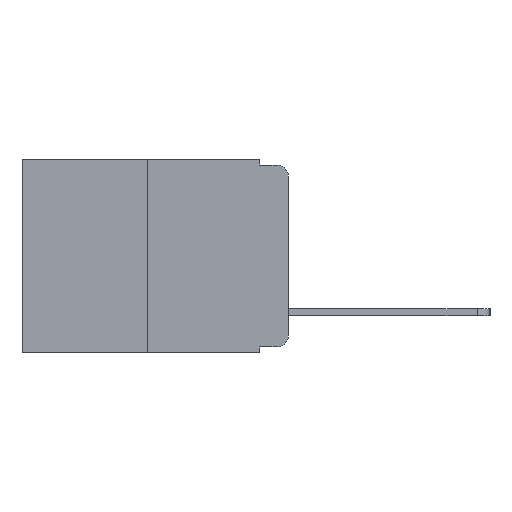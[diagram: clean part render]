
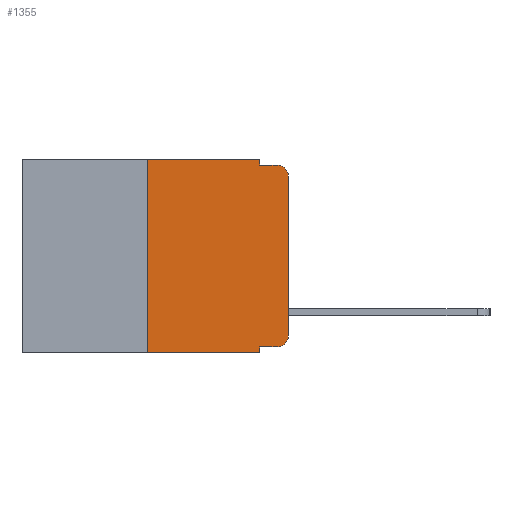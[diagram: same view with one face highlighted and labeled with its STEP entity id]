
A CAD part, left-side view. The second image highlights one B-rep face of the part: STEP entity #1355.
In plain terms, the highlighted planar face has unit normal (-1, 0, 0).
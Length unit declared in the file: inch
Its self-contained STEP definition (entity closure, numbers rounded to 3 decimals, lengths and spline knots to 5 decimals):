
#129 = CARTESIAN_POINT ( 'NONE',  ( 0., 0.051, -0.01 ) ) ;
#455 = VERTEX_POINT ( 'NONE', #19463 ) ;
#535 = CARTESIAN_POINT ( 'NONE',  ( 0., 0.051, 0. ) ) ;
#678 = CARTESIAN_POINT ( 'NONE',  ( 0., 0.25, 0. ) ) ;
#788 = CARTESIAN_POINT ( 'NONE',  ( 0., 0.02, -0.01 ) ) ;
#985 = AXIS2_PLACEMENT_3D ( 'NONE', #14498, #14367, #14458 ) ;
#998 = EDGE_CURVE ( 'NONE', #8953, #3451, #9735, .T. ) ;
#1194 = EDGE_CURVE ( 'NONE', #14783, #3736, #15493, .T. ) ;
#1355 = ADVANCED_FACE ( 'NONE', ( #13234 ), #6686, .F. ) ;
#1556 = VECTOR ( 'NONE', #4362, 39.37008 ) ;
#1994 = EDGE_CURVE ( 'NONE', #14861, #8953, #7348, .T. ) ;
#2044 = LINE ( 'NONE', #19117, #1556 ) ;
#3074 = LINE ( 'NONE', #5772, #10851 ) ;
#3287 = CIRCLE ( 'NONE', #14820, 0.02 ) ;
#3451 = VERTEX_POINT ( 'NONE', #788 ) ;
#3714 = CARTESIAN_POINT ( 'NONE',  ( 0., 0.473, -0.343 ) ) ;
#3736 = VERTEX_POINT ( 'NONE', #535 ) ;
#3832 = CARTESIAN_POINT ( 'NONE',  ( 0., 0.25, 0. ) ) ;
#3848 = VERTEX_POINT ( 'NONE', #13475 ) ;
#4027 = EDGE_CURVE ( 'NONE', #13659, #14783, #7723, .T. ) ;
#4066 = ORIENTED_EDGE ( 'NONE', *, *, #13524, .T. ) ;
#4362 = DIRECTION ( 'NONE',  ( 0., 0., -1. ) ) ;
#4597 = DIRECTION ( 'NONE',  ( -1., 0., 0. ) ) ;
#5683 = DIRECTION ( 'NONE',  ( 0., 0., 1. ) ) ;
#5772 = CARTESIAN_POINT ( 'NONE',  ( 0., 0.051, 0. ) ) ;
#6074 = ORIENTED_EDGE ( 'NONE', *, *, #18397, .F. ) ;
#6305 = VECTOR ( 'NONE', #12080, 39.37008 ) ;
#6686 = PLANE ( 'NONE',  #12114 ) ;
#6854 = VECTOR ( 'NONE', #5683, 39.37008 ) ;
#7272 = ORIENTED_EDGE ( 'NONE', *, *, #1194, .F. ) ;
#7284 = CARTESIAN_POINT ( 'NONE',  ( 0., 0., -0.313 ) ) ;
#7305 = LINE ( 'NONE', #14940, #6305 ) ;
#7348 = LINE ( 'NONE', #14639, #6854 ) ;
#7643 = CARTESIAN_POINT ( 'NONE',  ( 0., 0.051, -0.333 ) ) ;
#7723 = LINE ( 'NONE', #3832, #15604 ) ;
#8248 = CARTESIAN_POINT ( 'NONE',  ( 0., 0.473, 0. ) ) ;
#8554 = LINE ( 'NONE', #3714, #13025 ) ;
#8698 = CARTESIAN_POINT ( 'NONE',  ( 0., 0.25, -0.343 ) ) ;
#8895 = ORIENTED_EDGE ( 'NONE', *, *, #18286, .F. ) ;
#8952 = DIRECTION ( 'NONE',  ( 0., -1., 0. ) ) ;
#8953 = VERTEX_POINT ( 'NONE', #14530 ) ;
#9597 = ORIENTED_EDGE ( 'NONE', *, *, #1994, .T. ) ;
#9735 = CIRCLE ( 'NONE', #985, 0.02 ) ;
#10030 = CARTESIAN_POINT ( 'NONE',  ( 0., 0.473, 0. ) ) ;
#10629 = EDGE_CURVE ( 'NONE', #3848, #14861, #3287, .T. ) ;
#10851 = VECTOR ( 'NONE', #16196, 39.37008 ) ;
#11306 = DIRECTION ( 'NONE',  ( 1., 0., 0. ) ) ;
#11329 = DIRECTION ( 'NONE',  ( 0., 0., -1. ) ) ;
#11517 = ORIENTED_EDGE ( 'NONE', *, *, #10629, .T. ) ;
#11620 = VECTOR ( 'NONE', #14608, 39.37008 ) ;
#11870 = VECTOR ( 'NONE', #8952, 39.37008 ) ;
#12080 = DIRECTION ( 'NONE',  ( 0., -1., 0. ) ) ;
#12114 = AXIS2_PLACEMENT_3D ( 'NONE', #10030, #11306, #11329 ) ;
#13025 = VECTOR ( 'NONE', #14365, 39.37008 ) ;
#13234 = FACE_OUTER_BOUND ( 'NONE', #15201, .T. ) ;
#13475 = CARTESIAN_POINT ( 'NONE',  ( 0., 0.02, -0.333 ) ) ;
#13524 = EDGE_CURVE ( 'NONE', #13659, #455, #8554, .T. ) ;
#13659 = VERTEX_POINT ( 'NONE', #8698 ) ;
#13681 = CARTESIAN_POINT ( 'NONE',  ( 0., 0.02, -0.313 ) ) ;
#13754 = EDGE_CURVE ( 'NONE', #15208, #3451, #15719, .T. ) ;
#14365 = DIRECTION ( 'NONE',  ( 0., -1., 0. ) ) ;
#14367 = DIRECTION ( 'NONE',  ( -1., 0., 0. ) ) ;
#14403 = DIRECTION ( 'NONE',  ( 0., 0., 1. ) ) ;
#14458 = DIRECTION ( 'NONE',  ( 0., 0., -1. ) ) ;
#14498 = CARTESIAN_POINT ( 'NONE',  ( 0., 0.02, -0.03 ) ) ;
#14504 = ORIENTED_EDGE ( 'NONE', *, *, #15531, .T. ) ;
#14530 = CARTESIAN_POINT ( 'NONE',  ( 0., 0., -0.03 ) ) ;
#14608 = DIRECTION ( 'NONE',  ( 0., -1., 0. ) ) ;
#14639 = CARTESIAN_POINT ( 'NONE',  ( 0., 0., 0. ) ) ;
#14783 = VERTEX_POINT ( 'NONE', #678 ) ;
#14820 = AXIS2_PLACEMENT_3D ( 'NONE', #13681, #4597, #15128 ) ;
#14861 = VERTEX_POINT ( 'NONE', #7284 ) ;
#14940 = CARTESIAN_POINT ( 'NONE',  ( 0., 0.051, -0.333 ) ) ;
#15128 = DIRECTION ( 'NONE',  ( 0., 0., -1. ) ) ;
#15201 = EDGE_LOOP ( 'NONE', ( #9597, #17853, #19143, #8895, #7272, #15621, #4066, #6074, #14504, #11517 ) ) ;
#15208 = VERTEX_POINT ( 'NONE', #129 ) ;
#15493 = LINE ( 'NONE', #8248, #11620 ) ;
#15531 = EDGE_CURVE ( 'NONE', #18480, #3848, #7305, .T. ) ;
#15604 = VECTOR ( 'NONE', #14403, 39.37008 ) ;
#15621 = ORIENTED_EDGE ( 'NONE', *, *, #4027, .F. ) ;
#15719 = LINE ( 'NONE', #17759, #11870 ) ;
#16196 = DIRECTION ( 'NONE',  ( 0., 0., -1. ) ) ;
#17759 = CARTESIAN_POINT ( 'NONE',  ( 0., 0.051, -0.01 ) ) ;
#17853 = ORIENTED_EDGE ( 'NONE', *, *, #998, .T. ) ;
#18286 = EDGE_CURVE ( 'NONE', #3736, #15208, #3074, .T. ) ;
#18397 = EDGE_CURVE ( 'NONE', #18480, #455, #2044, .T. ) ;
#18480 = VERTEX_POINT ( 'NONE', #7643 ) ;
#19117 = CARTESIAN_POINT ( 'NONE',  ( 0., 0.051, 0. ) ) ;
#19143 = ORIENTED_EDGE ( 'NONE', *, *, #13754, .F. ) ;
#19463 = CARTESIAN_POINT ( 'NONE',  ( 0., 0.051, -0.343 ) ) ;
